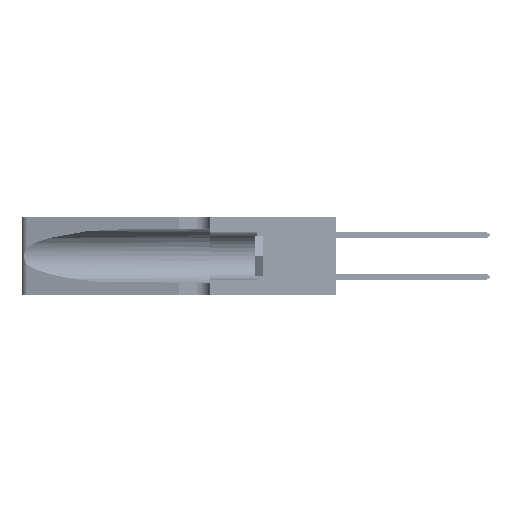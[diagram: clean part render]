
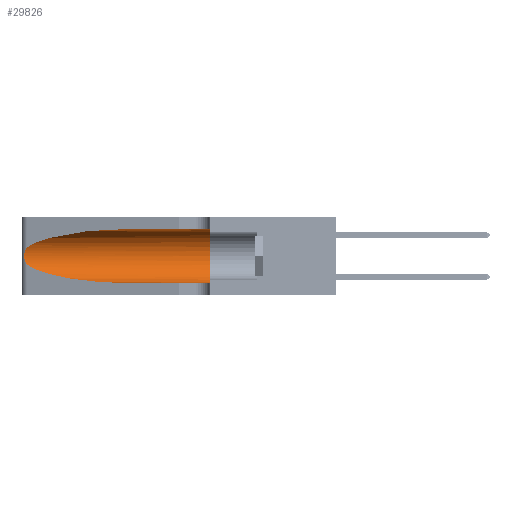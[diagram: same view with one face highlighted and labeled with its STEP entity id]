
A CAD part, left-side view. The second image highlights one B-rep face of the part: STEP entity #29826.
In plain terms, the highlighted cylindrical face has radius 3.308 mm (diameter 6.617 mm), a partial arc.
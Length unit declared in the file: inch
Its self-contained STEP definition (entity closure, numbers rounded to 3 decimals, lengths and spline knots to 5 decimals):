
#191 = VERTEX_POINT ( 'NONE', #10909 ) ;
#301 = DIRECTION ( 'NONE',  ( 0., 0., 1. ) ) ;
#380 = AXIS2_PLACEMENT_3D ( 'NONE', #46683, #23695, #301 ) ;
#387 = ORIENTED_EDGE ( 'NONE', *, *, #37683, .F. ) ;
#533 = AXIS2_PLACEMENT_3D ( 'NONE', #6289, #18033, #2310 ) ;
#670 = VERTEX_POINT ( 'NONE', #48073 ) ;
#1078 = EDGE_CURVE ( 'NONE', #20802, #670, #32546, .T. ) ;
#2239 = EDGE_LOOP ( 'NONE', ( #19848, #37989, #36469, #5467, #10308, #387 ) ) ;
#2279 = CARTESIAN_POINT ( 'NONE',  ( 0.2373, 1.15595, 0.08982 ) ) ;
#2310 = DIRECTION ( 'NONE',  ( 0., 0., -1. ) ) ;
#2702 = CARTESIAN_POINT ( 'NONE',  ( 0.25639, 1.23186, 0.15144 ) ) ;
#4004 = CYLINDRICAL_SURFACE ( 'NONE', #533, 0.13025 ) ;
#4360 = CARTESIAN_POINT ( 'NONE',  ( 0.1305, 0.72297, 0.05475 ) ) ;
#5102 = DIRECTION ( 'NONE',  ( 0., -1., 0. ) ) ;
#5233 = FACE_OUTER_BOUND ( 'NONE', #2239, .T. ) ;
#5467 = ORIENTED_EDGE ( 'NONE', *, *, #29596, .T. ) ;
#6289 = CARTESIAN_POINT ( 'NONE',  ( 0.1305, 1.61858, 0.185 ) ) ;
#6669 = CARTESIAN_POINT ( 'NONE',  ( 0.25487, 1.22718, 0.14631 ) ) ;
#7071 = CARTESIAN_POINT ( 'NONE',  ( 0.1305, 1.61858, 0.31525 ) ) ;
#7882 = CARTESIAN_POINT ( 'NONE',  ( 0.25487, 1.22718, 0.22369 ) ) ;
#10308 = ORIENTED_EDGE ( 'NONE', *, *, #12447, .F. ) ;
#10364 = EDGE_CURVE ( 'NONE', #670, #49766, #14565, .T. ) ;
#10909 = CARTESIAN_POINT ( 'NONE',  ( 0.1305, 0.72297, 0.31525 ) ) ;
#12447 = EDGE_CURVE ( 'NONE', #24944, #14088, #33920, .T. ) ;
#13403 = VECTOR ( 'NONE', #45531, 39.37008 ) ;
#14088 = VERTEX_POINT ( 'NONE', #27923 ) ;
#14095 = CARTESIAN_POINT ( 'NONE',  ( 0.1305, 0.72297, 0.31525 ) ) ;
#14117 = CARTESIAN_POINT ( 'NONE',  ( 0.18966, 0.96281, 0.05475 ) ) ;
#14565 =( BOUNDED_CURVE ( )  B_SPLINE_CURVE ( 3, ( #40928, #2279, #14117, #41079 ),
 .UNSPECIFIED., .F., .F. ) 
 B_SPLINE_CURVE_WITH_KNOTS ( ( 4, 4 ),
 ( 3.44316, 4.71239 ),
 .UNSPECIFIED. ) 
 CURVE ( )  GEOMETRIC_REPRESENTATION_ITEM ( )  RATIONAL_B_SPLINE_CURVE ( ( 1., 0.87, 0.87, 1. ) ) 
 REPRESENTATION_ITEM ( '' )  );
#18033 = DIRECTION ( 'NONE',  ( 0., -1., 0. ) ) ;
#18241 = CARTESIAN_POINT ( 'NONE',  ( 0.26075, 1.23896, 0.19203 ) ) ;
#19685 = CARTESIAN_POINT ( 'NONE',  ( 0.25555, 1.22994, 0.2215 ) ) ;
#19848 = ORIENTED_EDGE ( 'NONE', *, *, #28326, .T. ) ;
#19855 =( BOUNDED_CURVE ( )  B_SPLINE_CURVE ( 3, ( #14095, #37216, #48716, #25761 ),
 .UNSPECIFIED., .F., .F. ) 
 B_SPLINE_CURVE_WITH_KNOTS ( ( 4, 4 ),
 ( 1.5708, 2.84003 ),
 .UNSPECIFIED. ) 
 CURVE ( )  GEOMETRIC_REPRESENTATION_ITEM ( )  RATIONAL_B_SPLINE_CURVE ( ( 1., 0.87, 0.87, 1. ) ) 
 REPRESENTATION_ITEM ( '' )  );
#20600 = CARTESIAN_POINT ( 'NONE',  ( 0.1305, 1.61858, 0.05475 ) ) ;
#20802 = VERTEX_POINT ( 'NONE', #7882 ) ;
#21194 = CARTESIAN_POINT ( 'NONE',  ( 0.25787, 1.23484, 0.2124 ) ) ;
#22125 = CARTESIAN_POINT ( 'NONE',  ( 0.26017, 1.23833, 0.17102 ) ) ;
#23542 = CARTESIAN_POINT ( 'NONE',  ( 0.25487, 1.22718, 0.22369 ) ) ;
#23680 = LINE ( 'NONE', #7071, #13403 ) ;
#23695 = DIRECTION ( 'NONE',  ( 0., 1., 0. ) ) ;
#24944 = VERTEX_POINT ( 'NONE', #35759 ) ;
#25761 = CARTESIAN_POINT ( 'NONE',  ( 0.25487, 1.22718, 0.22369 ) ) ;
#25893 = CARTESIAN_POINT ( 'NONE',  ( 0.25854, 1.2359, 0.20912 ) ) ;
#26025 = CARTESIAN_POINT ( 'NONE',  ( 0.25789, 1.23486, 0.15765 ) ) ;
#27923 = CARTESIAN_POINT ( 'NONE',  ( 0.1305, 0.35, 0.05475 ) ) ;
#28326 = EDGE_CURVE ( 'NONE', #191, #20802, #19855, .T. ) ;
#29596 = EDGE_CURVE ( 'NONE', #49766, #14088, #46924, .T. ) ;
#29826 = ADVANCED_FACE ( 'NONE', ( #5233 ), #4004, .F. ) ;
#29927 = CARTESIAN_POINT ( 'NONE',  ( 0.25555, 1.22993, 0.14849 ) ) ;
#31347 = CARTESIAN_POINT ( 'NONE',  ( 0.25639, 1.23184, 0.21858 ) ) ;
#32546 = B_SPLINE_CURVE_WITH_KNOTS ( 'NONE', 3,
 ( #23542, #19685, #31347, #21194, #25893, #41309, #18241, #45145, #22125, #48960, #26025, #2702, #29927, #6669 ),
 .UNSPECIFIED., .F., .F.,
 ( 4, 2, 2, 2, 2, 2, 4 ),
 ( 0., 0.00027, 0.00053, 0.00107, 0.0016, 0.00187, 0.00214 ),
 .UNSPECIFIED. ) ;
#33920 = CIRCLE ( 'NONE', #380, 0.13025 ) ;
#35759 = CARTESIAN_POINT ( 'NONE',  ( 0.1305, 0.35, 0.31525 ) ) ;
#36469 = ORIENTED_EDGE ( 'NONE', *, *, #10364, .T. ) ;
#37216 = CARTESIAN_POINT ( 'NONE',  ( 0.18966, 0.96281, 0.31525 ) ) ;
#37683 = EDGE_CURVE ( 'NONE', #191, #24944, #23680, .T. ) ;
#37989 = ORIENTED_EDGE ( 'NONE', *, *, #1078, .T. ) ;
#40928 = CARTESIAN_POINT ( 'NONE',  ( 0.25487, 1.22718, 0.14631 ) ) ;
#41079 = CARTESIAN_POINT ( 'NONE',  ( 0.1305, 0.72297, 0.05475 ) ) ;
#41309 = CARTESIAN_POINT ( 'NONE',  ( 0.26018, 1.23835, 0.19895 ) ) ;
#45145 = CARTESIAN_POINT ( 'NONE',  ( 0.26075, 1.23896, 0.178 ) ) ;
#45531 = DIRECTION ( 'NONE',  ( 0., -1., 0. ) ) ;
#45745 = VECTOR ( 'NONE', #5102, 39.37008 ) ;
#46683 = CARTESIAN_POINT ( 'NONE',  ( 0.1305, 0.35, 0.185 ) ) ;
#46924 = LINE ( 'NONE', #20600, #45745 ) ;
#48073 = CARTESIAN_POINT ( 'NONE',  ( 0.25487, 1.22718, 0.14631 ) ) ;
#48716 = CARTESIAN_POINT ( 'NONE',  ( 0.2373, 1.15595, 0.28018 ) ) ;
#48960 = CARTESIAN_POINT ( 'NONE',  ( 0.25856, 1.23593, 0.16098 ) ) ;
#49766 = VERTEX_POINT ( 'NONE', #4360 ) ;
